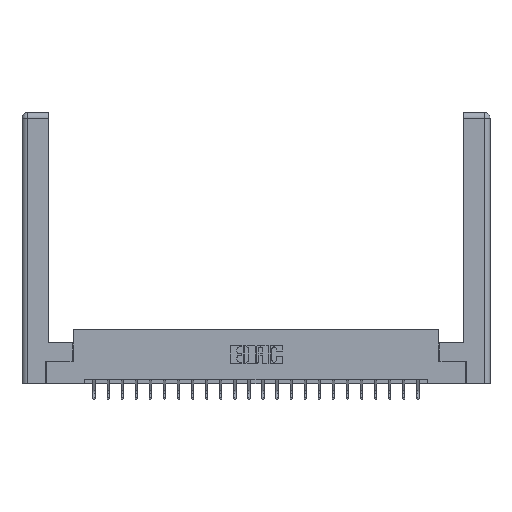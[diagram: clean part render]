
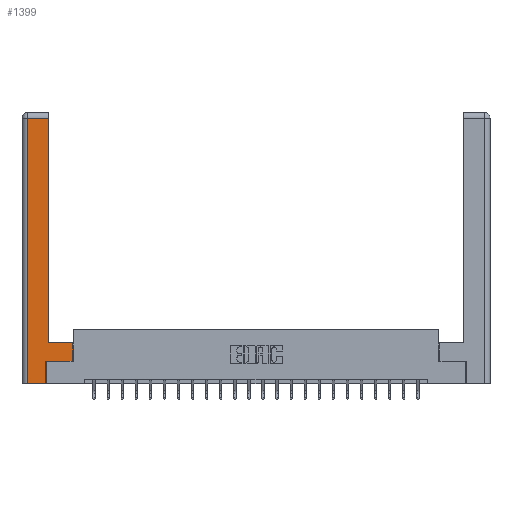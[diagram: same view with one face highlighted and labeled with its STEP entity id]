
A CAD part, top view. The second image highlights one B-rep face of the part: STEP entity #1399.
In plain terms, the highlighted planar face has unit normal (0, 0, 1).
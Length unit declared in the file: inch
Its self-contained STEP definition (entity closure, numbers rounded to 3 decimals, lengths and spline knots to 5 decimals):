
#174 = VECTOR ( 'NONE', #15821, 39.37008 ) ;
#186 = LINE ( 'NONE', #6606, #7165 ) ;
#709 = CARTESIAN_POINT ( 'NONE',  ( 0.0615, 0., 0. ) ) ;
#727 = EDGE_CURVE ( 'NONE', #13015, #4299, #10195, .T. ) ;
#1221 = DIRECTION ( 'NONE',  ( -1., 0., 0. ) ) ;
#1303 = CARTESIAN_POINT ( 'NONE',  ( 0.295, 0.45, 0. ) ) ;
#1374 = VECTOR ( 'NONE', #6879, 39.37008 ) ;
#1399 = ADVANCED_FACE ( 'NONE', ( #13321 ), #7073, .F. ) ;
#4098 = LINE ( 'NONE', #9061, #6126 ) ;
#4149 = EDGE_CURVE ( 'NONE', #22339, #15370, #17160, .T. ) ;
#4299 = VERTEX_POINT ( 'NONE', #18822 ) ;
#5479 = CARTESIAN_POINT ( 'NONE',  ( 0.565, 0.245, 0. ) ) ;
#6126 = VECTOR ( 'NONE', #16610, 39.37008 ) ;
#6529 = VERTEX_POINT ( 'NONE', #709 ) ;
#6606 = CARTESIAN_POINT ( 'NONE',  ( 0.265, 0., 0. ) ) ;
#6679 = VERTEX_POINT ( 'NONE', #17995 ) ;
#6879 = DIRECTION ( 'NONE',  ( 0., 1., 0. ) ) ;
#7073 = PLANE ( 'NONE',  #10803 ) ;
#7165 = VECTOR ( 'NONE', #12033, 39.37008 ) ;
#7634 = VECTOR ( 'NONE', #1221, 39.37008 ) ;
#8195 = DIRECTION ( 'NONE',  ( -1., 0., 0. ) ) ;
#8462 = CARTESIAN_POINT ( 'NONE',  ( 0.265, 0.245, 0. ) ) ;
#8568 = ORIENTED_EDGE ( 'NONE', *, *, #16636, .T. ) ;
#9061 = CARTESIAN_POINT ( 'NONE',  ( 0.565, 0.245, 0. ) ) ;
#9189 = ORIENTED_EDGE ( 'NONE', *, *, #12437, .T. ) ;
#10195 = LINE ( 'NONE', #8462, #12174 ) ;
#10314 = DIRECTION ( 'NONE',  ( 0., 1., 0. ) ) ;
#10709 = DIRECTION ( 'NONE',  ( 0., 0., -1. ) ) ;
#10803 = AXIS2_PLACEMENT_3D ( 'NONE', #19775, #10709, #8195 ) ;
#10959 = EDGE_CURVE ( 'NONE', #15370, #12058, #14226, .T. ) ;
#10965 = ORIENTED_EDGE ( 'NONE', *, *, #11979, .T. ) ;
#10980 = VECTOR ( 'NONE', #11702, 39.37008 ) ;
#11283 = EDGE_CURVE ( 'NONE', #6679, #6529, #18664, .T. ) ;
#11702 = DIRECTION ( 'NONE',  ( 0., -1., 0. ) ) ;
#11979 = EDGE_CURVE ( 'NONE', #12058, #14512, #18047, .T. ) ;
#12033 = DIRECTION ( 'NONE',  ( 1., 0., 0. ) ) ;
#12058 = VERTEX_POINT ( 'NONE', #23282 ) ;
#12174 = VECTOR ( 'NONE', #10314, 39.37008 ) ;
#12437 = EDGE_CURVE ( 'NONE', #6529, #13015, #186, .T. ) ;
#12456 = CARTESIAN_POINT ( 'NONE',  ( 0.565, 0.45, 0. ) ) ;
#13015 = VERTEX_POINT ( 'NONE', #19276 ) ;
#13321 = FACE_OUTER_BOUND ( 'NONE', #14167, .T. ) ;
#13702 = CARTESIAN_POINT ( 'NONE',  ( 0.0615, 0., 0. ) ) ;
#14167 = EDGE_LOOP ( 'NONE', ( #10965, #15420, #14529, #9189, #21002, #8568, #22450, #15481 ) ) ;
#14226 = LINE ( 'NONE', #1303, #7634 ) ;
#14512 = VERTEX_POINT ( 'NONE', #19448 ) ;
#14529 = ORIENTED_EDGE ( 'NONE', *, *, #11283, .T. ) ;
#14570 = LINE ( 'NONE', #18115, #17670 ) ;
#15370 = VERTEX_POINT ( 'NONE', #12456 ) ;
#15420 = ORIENTED_EDGE ( 'NONE', *, *, #20682, .T. ) ;
#15481 = ORIENTED_EDGE ( 'NONE', *, *, #10959, .T. ) ;
#15821 = DIRECTION ( 'NONE',  ( 0., 1., 0. ) ) ;
#16610 = DIRECTION ( 'NONE',  ( 1., 0., 0. ) ) ;
#16636 = EDGE_CURVE ( 'NONE', #4299, #22339, #4098, .T. ) ;
#17160 = LINE ( 'NONE', #21245, #174 ) ;
#17670 = VECTOR ( 'NONE', #21730, 39.37008 ) ;
#17720 = CARTESIAN_POINT ( 'NONE',  ( 0.295, 3., 0. ) ) ;
#17995 = CARTESIAN_POINT ( 'NONE',  ( 0.0615, 2.94, 0. ) ) ;
#18047 = LINE ( 'NONE', #17720, #1374 ) ;
#18115 = CARTESIAN_POINT ( 'NONE',  ( 0.0615, 2.94, 0. ) ) ;
#18664 = LINE ( 'NONE', #13702, #10980 ) ;
#18822 = CARTESIAN_POINT ( 'NONE',  ( 0.265, 0.245, 0. ) ) ;
#19276 = CARTESIAN_POINT ( 'NONE',  ( 0.265, 0., 0. ) ) ;
#19448 = CARTESIAN_POINT ( 'NONE',  ( 0.295, 2.94, 0. ) ) ;
#19775 = CARTESIAN_POINT ( 'NONE',  ( 0., 0., 0. ) ) ;
#20682 = EDGE_CURVE ( 'NONE', #14512, #6679, #14570, .T. ) ;
#21002 = ORIENTED_EDGE ( 'NONE', *, *, #727, .T. ) ;
#21245 = CARTESIAN_POINT ( 'NONE',  ( 0.565, 0.45, 0. ) ) ;
#21730 = DIRECTION ( 'NONE',  ( -1., 0., 0. ) ) ;
#22339 = VERTEX_POINT ( 'NONE', #5479 ) ;
#22450 = ORIENTED_EDGE ( 'NONE', *, *, #4149, .T. ) ;
#23282 = CARTESIAN_POINT ( 'NONE',  ( 0.295, 0.45, 0. ) ) ;
